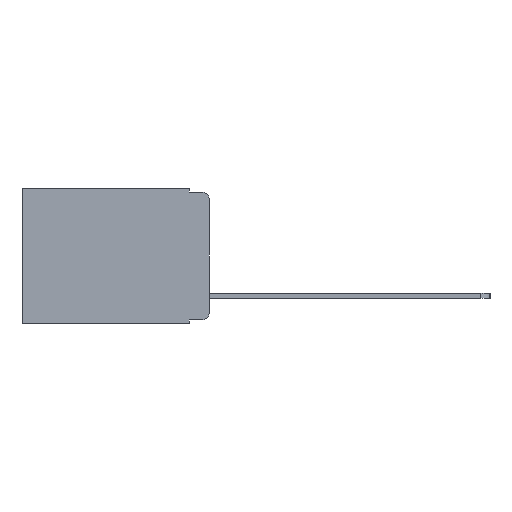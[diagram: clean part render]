
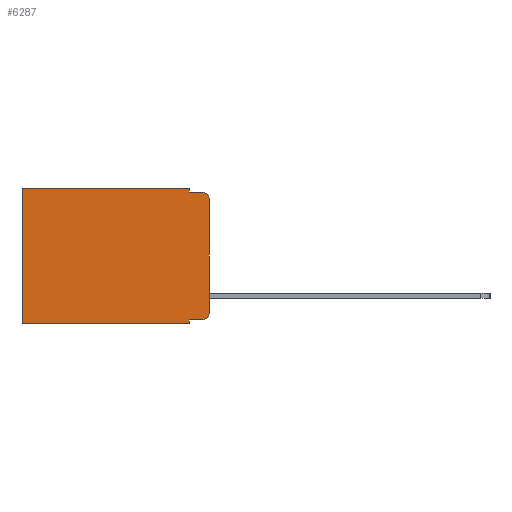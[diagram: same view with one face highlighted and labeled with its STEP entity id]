
A CAD part, left-side view. The second image highlights one B-rep face of the part: STEP entity #6287.
In plain terms, the highlighted planar face has unit normal (-1, 0, 0).
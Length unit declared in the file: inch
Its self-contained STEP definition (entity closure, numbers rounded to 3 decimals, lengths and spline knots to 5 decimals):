
#280 = VECTOR ( 'NONE', #13094, 39.37008 ) ;
#658 = VERTEX_POINT ( 'NONE', #13845 ) ;
#675 = ORIENTED_EDGE ( 'NONE', *, *, #14737, .F. ) ;
#685 = VECTOR ( 'NONE', #18664, 39.37008 ) ;
#1085 = CIRCLE ( 'NONE', #5756, 0.02 ) ;
#1137 = CIRCLE ( 'NONE', #5700, 0.02 ) ;
#1357 = DIRECTION ( 'NONE',  ( -1., 0., 0. ) ) ;
#1452 = ORIENTED_EDGE ( 'NONE', *, *, #12595, .T. ) ;
#1549 = VECTOR ( 'NONE', #13467, 39.37008 ) ;
#1607 = LINE ( 'NONE', #1939, #9358 ) ;
#1939 = CARTESIAN_POINT ( 'NONE',  ( 0.298, 0., 0. ) ) ;
#2685 = EDGE_CURVE ( 'NONE', #16969, #3760, #18373, .T. ) ;
#2686 = VECTOR ( 'NONE', #10570, 39.37008 ) ;
#2807 = CARTESIAN_POINT ( 'NONE',  ( 0.298, 0.02, -0.313 ) ) ;
#2898 = CARTESIAN_POINT ( 'NONE',  ( 0.298, 0.473, 0. ) ) ;
#3078 = CARTESIAN_POINT ( 'NONE',  ( 0.298, 0.051, 0. ) ) ;
#3143 = ORIENTED_EDGE ( 'NONE', *, *, #11851, .F. ) ;
#3598 = VERTEX_POINT ( 'NONE', #9906 ) ;
#3697 = ORIENTED_EDGE ( 'NONE', *, *, #13475, .F. ) ;
#3760 = VERTEX_POINT ( 'NONE', #15338 ) ;
#3856 = ORIENTED_EDGE ( 'NONE', *, *, #11703, .T. ) ;
#4304 = VERTEX_POINT ( 'NONE', #2898 ) ;
#4430 = DIRECTION ( 'NONE',  ( 0., 0., -1. ) ) ;
#4435 = CARTESIAN_POINT ( 'NONE',  ( 0.298, 0., 0. ) ) ;
#4523 = LINE ( 'NONE', #7067, #280 ) ;
#4606 = CARTESIAN_POINT ( 'NONE',  ( 0.298, 0.051, -0.343 ) ) ;
#4918 = LINE ( 'NONE', #13028, #685 ) ;
#4977 = LINE ( 'NONE', #17284, #12533 ) ;
#5352 = ORIENTED_EDGE ( 'NONE', *, *, #2685, .T. ) ;
#5562 = CARTESIAN_POINT ( 'NONE',  ( 0.298, 0., 0. ) ) ;
#5700 = AXIS2_PLACEMENT_3D ( 'NONE', #2807, #13464, #4430 ) ;
#5756 = AXIS2_PLACEMENT_3D ( 'NONE', #10620, #1357, #12121 ) ;
#6006 = VERTEX_POINT ( 'NONE', #8290 ) ;
#6287 = ADVANCED_FACE ( 'NONE', ( #13639 ), #15974, .F. ) ;
#6992 = CARTESIAN_POINT ( 'NONE',  ( 0.298, 0.051, -0.333 ) ) ;
#7005 = ORIENTED_EDGE ( 'NONE', *, *, #17572, .T. ) ;
#7067 = CARTESIAN_POINT ( 'NONE',  ( 0.298, 0.051, 0. ) ) ;
#7151 = DIRECTION ( 'NONE',  ( 1., 0., 0. ) ) ;
#7920 = EDGE_CURVE ( 'NONE', #16969, #18342, #4523, .T. ) ;
#8063 = EDGE_CURVE ( 'NONE', #3598, #6006, #17018, .T. ) ;
#8290 = CARTESIAN_POINT ( 'NONE',  ( 0.298, 0., -0.313 ) ) ;
#9358 = VECTOR ( 'NONE', #12015, 39.37008 ) ;
#9464 = VERTEX_POINT ( 'NONE', #13287 ) ;
#9534 = CARTESIAN_POINT ( 'NONE',  ( 0.298, 0.051, 0. ) ) ;
#9906 = CARTESIAN_POINT ( 'NONE',  ( 0.298, 0., -0.03 ) ) ;
#9940 = EDGE_CURVE ( 'NONE', #4304, #658, #14757, .T. ) ;
#10403 = ORIENTED_EDGE ( 'NONE', *, *, #9940, .T. ) ;
#10570 = DIRECTION ( 'NONE',  ( 0., 0., -1. ) ) ;
#10620 = CARTESIAN_POINT ( 'NONE',  ( 0.298, 0.02, -0.03 ) ) ;
#11703 = EDGE_CURVE ( 'NONE', #3760, #6006, #1137, .T. ) ;
#11851 = EDGE_CURVE ( 'NONE', #13836, #12380, #17753, .T. ) ;
#12015 = DIRECTION ( 'NONE',  ( 0., 1., 0. ) ) ;
#12121 = DIRECTION ( 'NONE',  ( 0., 0., -1. ) ) ;
#12380 = VERTEX_POINT ( 'NONE', #19057 ) ;
#12407 = DIRECTION ( 'NONE',  ( 0., -1., 0. ) ) ;
#12528 = EDGE_LOOP ( 'NONE', ( #15598, #7005, #675, #3143, #1452, #10403, #3697, #12862, #5352, #3856 ) ) ;
#12533 = VECTOR ( 'NONE', #18647, 39.37008 ) ;
#12595 = EDGE_CURVE ( 'NONE', #13836, #4304, #1607, .T. ) ;
#12793 = AXIS2_PLACEMENT_3D ( 'NONE', #5562, #7151, #17389 ) ;
#12862 = ORIENTED_EDGE ( 'NONE', *, *, #7920, .F. ) ;
#13028 = CARTESIAN_POINT ( 'NONE',  ( 0.298, 0.051, -0.01 ) ) ;
#13094 = DIRECTION ( 'NONE',  ( 0., 0., -1. ) ) ;
#13287 = CARTESIAN_POINT ( 'NONE',  ( 0.298, 0.02, -0.01 ) ) ;
#13464 = DIRECTION ( 'NONE',  ( -1., 0., 0. ) ) ;
#13467 = DIRECTION ( 'NONE',  ( 0., 0., -1. ) ) ;
#13475 = EDGE_CURVE ( 'NONE', #18342, #658, #4977, .T. ) ;
#13639 = FACE_OUTER_BOUND ( 'NONE', #12528, .T. ) ;
#13836 = VERTEX_POINT ( 'NONE', #9534 ) ;
#13842 = CARTESIAN_POINT ( 'NONE',  ( 0.298, 0.051, -0.333 ) ) ;
#13845 = CARTESIAN_POINT ( 'NONE',  ( 0.298, 0.473, -0.343 ) ) ;
#13998 = VECTOR ( 'NONE', #19316, 39.37008 ) ;
#14665 = VECTOR ( 'NONE', #12407, 39.37008 ) ;
#14737 = EDGE_CURVE ( 'NONE', #12380, #9464, #4918, .T. ) ;
#14757 = LINE ( 'NONE', #17783, #2686 ) ;
#15338 = CARTESIAN_POINT ( 'NONE',  ( 0.298, 0.02, -0.333 ) ) ;
#15598 = ORIENTED_EDGE ( 'NONE', *, *, #8063, .F. ) ;
#15974 = PLANE ( 'NONE',  #12793 ) ;
#16969 = VERTEX_POINT ( 'NONE', #13842 ) ;
#17018 = LINE ( 'NONE', #4435, #1549 ) ;
#17284 = CARTESIAN_POINT ( 'NONE',  ( 0.298, 0., -0.343 ) ) ;
#17389 = DIRECTION ( 'NONE',  ( 0., 0., -1. ) ) ;
#17572 = EDGE_CURVE ( 'NONE', #3598, #9464, #1085, .T. ) ;
#17753 = LINE ( 'NONE', #3078, #13998 ) ;
#17783 = CARTESIAN_POINT ( 'NONE',  ( 0.298, 0.473, 0. ) ) ;
#18342 = VERTEX_POINT ( 'NONE', #4606 ) ;
#18373 = LINE ( 'NONE', #6992, #14665 ) ;
#18647 = DIRECTION ( 'NONE',  ( 0., 1., 0. ) ) ;
#18664 = DIRECTION ( 'NONE',  ( 0., -1., 0. ) ) ;
#19057 = CARTESIAN_POINT ( 'NONE',  ( 0.298, 0.051, -0.01 ) ) ;
#19316 = DIRECTION ( 'NONE',  ( 0., 0., -1. ) ) ;
